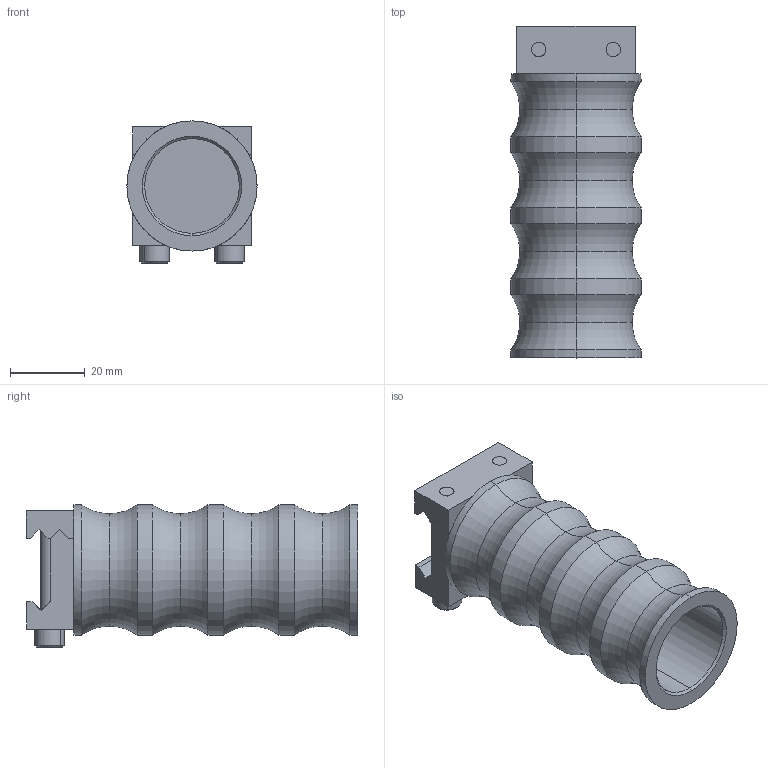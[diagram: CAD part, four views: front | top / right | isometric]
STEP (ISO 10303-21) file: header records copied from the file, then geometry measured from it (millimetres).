
FILE_DESCRIPTION (( 'STEP AP214' ), '1' );
FILE_NAME ('ForeGrip.STEP', '2015-01-24T03:30:16', ( 'WarFairy' ), ( '' ), 'SwSTEP 2.0', 'SolidWorks 2013', '' );
FILE_SCHEMA (( 'AUTOMOTIVE_DESIGN' ));
Length unit declared in the file: inch
Products named in the file (4): socket head cap screw_ai_HX-SHCS 0.19-32x1.25x0.875-N; ForeGrip-Retainer; ForeGrip
Assembly tree (4 placements, depth 2):
  ForeGrip
    ForeGrip
    ForeGrip-Retainer
    socket head cap screw_ai_HX-SHCS 0.19-32x1.25x0.875-N  x2
Bounding box: 34.92 x 89.03 x 38.16 mm (x, y, z)
Volume: 37435.8 mm3; surface area: 20420.8 mm2
Topology: 4 solids, 4 shells, 135 faces, 318 edges, 188 vertices
Faces by surface type: plane 69, cylinder 28, torus 20, cone 18
Entity records: 3344 total; most frequent: CARTESIAN_POINT 576, DIRECTION 572, ORIENTED_EDGE 516, EDGE_CURVE 258, AXIS2_PLACEMENT_3D 215, VERTEX_POINT 155, LINE 142, VECTOR 142
